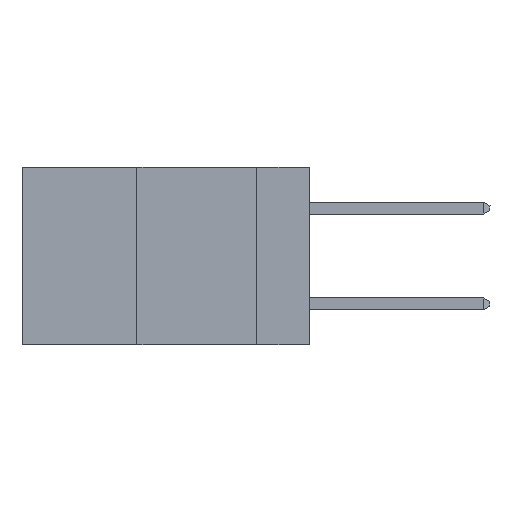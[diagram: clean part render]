
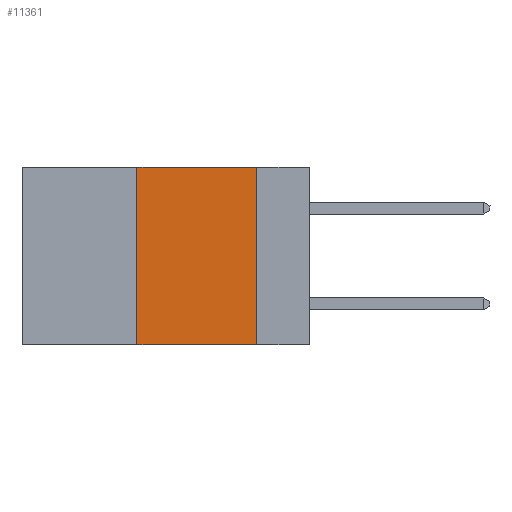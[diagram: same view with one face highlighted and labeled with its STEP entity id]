
A CAD part, left-side view. The second image highlights one B-rep face of the part: STEP entity #11361.
In plain terms, the highlighted planar face has unit normal (-1, 0, 0).
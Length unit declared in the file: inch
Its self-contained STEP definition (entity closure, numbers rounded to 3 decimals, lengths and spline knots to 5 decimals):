
#364 = AXIS2_PLACEMENT_3D ( 'NONE', #7680, #2454, #8565 ) ;
#654 = CARTESIAN_POINT ( 'NONE',  ( 0., 0.36, 0. ) ) ;
#870 = VERTEX_POINT ( 'NONE', #654 ) ;
#1060 = DIRECTION ( 'NONE',  ( 0., 0., -1. ) ) ;
#1647 = CARTESIAN_POINT ( 'NONE',  ( 0., 0.11, 0. ) ) ;
#1970 = CARTESIAN_POINT ( 'NONE',  ( 0., 0.36, -0.37 ) ) ;
#2454 = DIRECTION ( 'NONE',  ( 1., 0., 0. ) ) ;
#2819 = LINE ( 'NONE', #4938, #4892 ) ;
#3013 = CARTESIAN_POINT ( 'NONE',  ( 0., 0.36, 0. ) ) ;
#3397 = LINE ( 'NONE', #4009, #5460 ) ;
#3555 = VERTEX_POINT ( 'NONE', #1970 ) ;
#3968 = LINE ( 'NONE', #11545, #8520 ) ;
#4009 = CARTESIAN_POINT ( 'NONE',  ( 0., 0.6, -0.37 ) ) ;
#4892 = VECTOR ( 'NONE', #5814, 39.37008 ) ;
#4938 = CARTESIAN_POINT ( 'NONE',  ( 0., 0.6, 0. ) ) ;
#5460 = VECTOR ( 'NONE', #10841, 39.37008 ) ;
#5465 = ORIENTED_EDGE ( 'NONE', *, *, #9757, .F. ) ;
#5563 = ORIENTED_EDGE ( 'NONE', *, *, #9989, .F. ) ;
#5617 = ORIENTED_EDGE ( 'NONE', *, *, #9771, .F. ) ;
#5637 = ORIENTED_EDGE ( 'NONE', *, *, #9900, .T. ) ;
#5704 = FACE_OUTER_BOUND ( 'NONE', #8975, .T. ) ;
#5814 = DIRECTION ( 'NONE',  ( 0., -1., 0. ) ) ;
#6036 = VERTEX_POINT ( 'NONE', #6102 ) ;
#6063 = VERTEX_POINT ( 'NONE', #1647 ) ;
#6102 = CARTESIAN_POINT ( 'NONE',  ( 0., 0.11, -0.37 ) ) ;
#7325 = DIRECTION ( 'NONE',  ( 0., 0., 1. ) ) ;
#7680 = CARTESIAN_POINT ( 'NONE',  ( 0., 0.6, 0. ) ) ;
#8205 = LINE ( 'NONE', #3013, #10265 ) ;
#8520 = VECTOR ( 'NONE', #1060, 39.37008 ) ;
#8565 = DIRECTION ( 'NONE',  ( 0., 0., -1. ) ) ;
#8975 = EDGE_LOOP ( 'NONE', ( #5465, #5563, #5617, #5637 ) ) ;
#9757 = EDGE_CURVE ( 'NONE', #6063, #6036, #3968, .T. ) ;
#9771 = EDGE_CURVE ( 'NONE', #3555, #870, #8205, .T. ) ;
#9900 = EDGE_CURVE ( 'NONE', #3555, #6036, #3397, .T. ) ;
#9989 = EDGE_CURVE ( 'NONE', #870, #6063, #2819, .T. ) ;
#10251 = PLANE ( 'NONE',  #364 ) ;
#10265 = VECTOR ( 'NONE', #7325, 39.37008 ) ;
#10841 = DIRECTION ( 'NONE',  ( 0., -1., 0. ) ) ;
#11361 = ADVANCED_FACE ( 'NONE', ( #5704 ), #10251, .F. ) ;
#11545 = CARTESIAN_POINT ( 'NONE',  ( 0., 0.11, 0. ) ) ;
